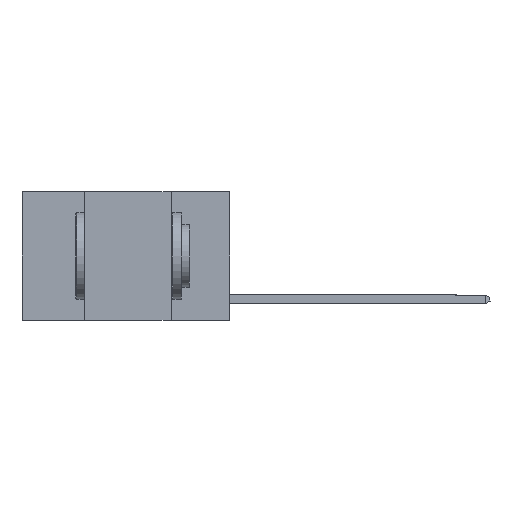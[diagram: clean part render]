
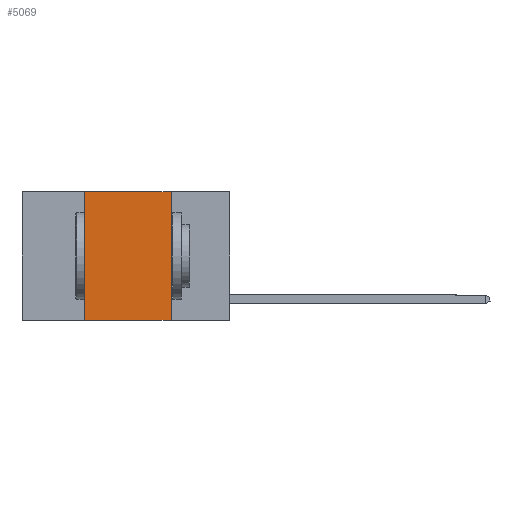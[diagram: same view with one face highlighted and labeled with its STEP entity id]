
A CAD part, left-side view. The second image highlights one B-rep face of the part: STEP entity #5069.
In plain terms, the highlighted planar face has unit normal (-1, 0, 0).
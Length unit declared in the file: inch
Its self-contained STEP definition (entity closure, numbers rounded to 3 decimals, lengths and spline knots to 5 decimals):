
#723 = AXIS2_PLACEMENT_3D ( 'NONE', #9114, #13439, #6968 ) ;
#728 = VECTOR ( 'NONE', #13632, 39.37008 ) ;
#844 = VECTOR ( 'NONE', #4097, 39.37008 ) ;
#1435 = EDGE_CURVE ( 'NONE', #6226, #2001, #12424, .T. ) ;
#2001 = VERTEX_POINT ( 'NONE', #13237 ) ;
#2447 = ORIENTED_EDGE ( 'NONE', *, *, #3652, .F. ) ;
#2846 = LINE ( 'NONE', #5341, #9751 ) ;
#3544 = CARTESIAN_POINT ( 'NONE',  ( 0., 0.17, 0. ) ) ;
#3652 = EDGE_CURVE ( 'NONE', #9612, #8329, #6099, .T. ) ;
#3817 = DIRECTION ( 'NONE',  ( 0., 0., -1. ) ) ;
#4097 = DIRECTION ( 'NONE',  ( 0., -1., 0. ) ) ;
#4931 = EDGE_LOOP ( 'NONE', ( #9017, #2447, #5356, #8864 ) ) ;
#5069 = ADVANCED_FACE ( 'NONE', ( #12516 ), #11280, .F. ) ;
#5302 = CARTESIAN_POINT ( 'NONE',  ( 0., 0.6, 0. ) ) ;
#5341 = CARTESIAN_POINT ( 'NONE',  ( 0., 0.42, 0. ) ) ;
#5356 = ORIENTED_EDGE ( 'NONE', *, *, #8074, .F. ) ;
#6099 = LINE ( 'NONE', #5302, #844 ) ;
#6226 = VERTEX_POINT ( 'NONE', #12283 ) ;
#6968 = DIRECTION ( 'NONE',  ( 0., 0., -1. ) ) ;
#7790 = LINE ( 'NONE', #10376, #8801 ) ;
#8074 = EDGE_CURVE ( 'NONE', #6226, #9612, #2846, .T. ) ;
#8329 = VERTEX_POINT ( 'NONE', #3544 ) ;
#8801 = VECTOR ( 'NONE', #3817, 39.37008 ) ;
#8864 = ORIENTED_EDGE ( 'NONE', *, *, #1435, .T. ) ;
#9017 = ORIENTED_EDGE ( 'NONE', *, *, #11606, .F. ) ;
#9114 = CARTESIAN_POINT ( 'NONE',  ( 0., 0.6, 0. ) ) ;
#9612 = VERTEX_POINT ( 'NONE', #10099 ) ;
#9751 = VECTOR ( 'NONE', #14040, 39.37008 ) ;
#10099 = CARTESIAN_POINT ( 'NONE',  ( 0., 0.42, 0. ) ) ;
#10376 = CARTESIAN_POINT ( 'NONE',  ( 0., 0.17, 0. ) ) ;
#10909 = CARTESIAN_POINT ( 'NONE',  ( 0., 0.6, -0.37 ) ) ;
#11280 = PLANE ( 'NONE',  #723 ) ;
#11606 = EDGE_CURVE ( 'NONE', #8329, #2001, #7790, .T. ) ;
#12283 = CARTESIAN_POINT ( 'NONE',  ( 0., 0.42, -0.37 ) ) ;
#12424 = LINE ( 'NONE', #10909, #728 ) ;
#12516 = FACE_OUTER_BOUND ( 'NONE', #4931, .T. ) ;
#13237 = CARTESIAN_POINT ( 'NONE',  ( 0., 0.17, -0.37 ) ) ;
#13439 = DIRECTION ( 'NONE',  ( 1., 0., 0. ) ) ;
#13632 = DIRECTION ( 'NONE',  ( 0., -1., 0. ) ) ;
#14040 = DIRECTION ( 'NONE',  ( 0., 0., 1. ) ) ;
